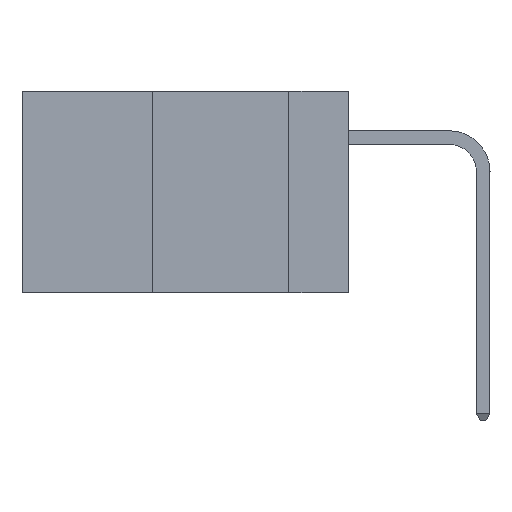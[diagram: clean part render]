
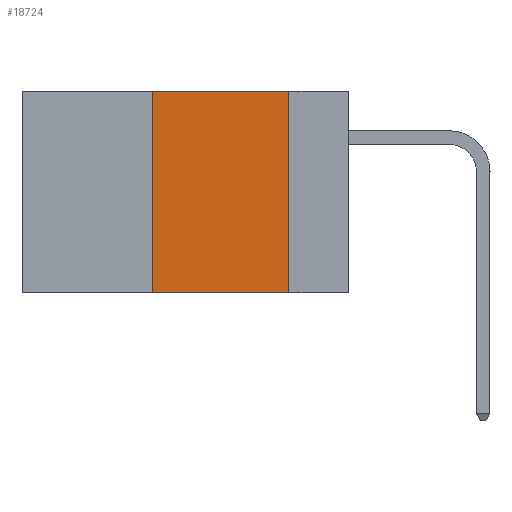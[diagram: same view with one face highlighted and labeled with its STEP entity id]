
A CAD part, left-side view. The second image highlights one B-rep face of the part: STEP entity #18724.
In plain terms, the highlighted planar face has unit normal (-1, 0, 0).
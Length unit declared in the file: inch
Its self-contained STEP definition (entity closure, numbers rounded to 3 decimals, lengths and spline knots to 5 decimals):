
#176 = EDGE_CURVE ( 'NONE', #11335, #14399, #16615, .T. ) ;
#1386 = CARTESIAN_POINT ( 'NONE',  ( 0., 0.6, 0. ) ) ;
#3761 = LINE ( 'NONE', #10688, #16018 ) ;
#4529 = CARTESIAN_POINT ( 'NONE',  ( 0., 0.36, 0. ) ) ;
#4796 = PLANE ( 'NONE',  #18789 ) ;
#5368 = VECTOR ( 'NONE', #12173, 39.37008 ) ;
#5467 = CARTESIAN_POINT ( 'NONE',  ( 0., 0.6, 0. ) ) ;
#6201 = CARTESIAN_POINT ( 'NONE',  ( 0., 0.36, 0. ) ) ;
#6330 = VECTOR ( 'NONE', #13210, 39.37008 ) ;
#7177 = CARTESIAN_POINT ( 'NONE',  ( 0., 0.11, 0. ) ) ;
#8136 = EDGE_CURVE ( 'NONE', #11138, #11335, #15712, .T. ) ;
#8621 = CARTESIAN_POINT ( 'NONE',  ( 0., 0.36, -0.37 ) ) ;
#9124 = CARTESIAN_POINT ( 'NONE',  ( 0., 0.11, -0.37 ) ) ;
#9139 = DIRECTION ( 'NONE',  ( 0., -1., 0. ) ) ;
#9486 = DIRECTION ( 'NONE',  ( 0., 0., 1. ) ) ;
#9931 = EDGE_CURVE ( 'NONE', #17806, #11138, #20955, .T. ) ;
#10688 = CARTESIAN_POINT ( 'NONE',  ( 0., 0.6, -0.37 ) ) ;
#11121 = VECTOR ( 'NONE', #9486, 39.37008 ) ;
#11138 = VERTEX_POINT ( 'NONE', #4529 ) ;
#11315 = EDGE_CURVE ( 'NONE', #17806, #14399, #3761, .T. ) ;
#11335 = VERTEX_POINT ( 'NONE', #7177 ) ;
#11443 = CARTESIAN_POINT ( 'NONE',  ( 0., 0.11, 0. ) ) ;
#11721 = FACE_OUTER_BOUND ( 'NONE', #14559, .T. ) ;
#12173 = DIRECTION ( 'NONE',  ( 0., -1., 0. ) ) ;
#12802 = ORIENTED_EDGE ( 'NONE', *, *, #8136, .F. ) ;
#13210 = DIRECTION ( 'NONE',  ( 0., 0., -1. ) ) ;
#14399 = VERTEX_POINT ( 'NONE', #9124 ) ;
#14559 = EDGE_LOOP ( 'NONE', ( #19497, #12802, #18206, #18069 ) ) ;
#15032 = DIRECTION ( 'NONE',  ( 0., 0., -1. ) ) ;
#15712 = LINE ( 'NONE', #5467, #5368 ) ;
#16018 = VECTOR ( 'NONE', #9139, 39.37008 ) ;
#16615 = LINE ( 'NONE', #11443, #6330 ) ;
#16680 = DIRECTION ( 'NONE',  ( 1., 0., 0. ) ) ;
#17806 = VERTEX_POINT ( 'NONE', #8621 ) ;
#18069 = ORIENTED_EDGE ( 'NONE', *, *, #11315, .T. ) ;
#18206 = ORIENTED_EDGE ( 'NONE', *, *, #9931, .F. ) ;
#18724 = ADVANCED_FACE ( 'NONE', ( #11721 ), #4796, .F. ) ;
#18789 = AXIS2_PLACEMENT_3D ( 'NONE', #1386, #16680, #15032 ) ;
#19497 = ORIENTED_EDGE ( 'NONE', *, *, #176, .F. ) ;
#20955 = LINE ( 'NONE', #6201, #11121 ) ;
